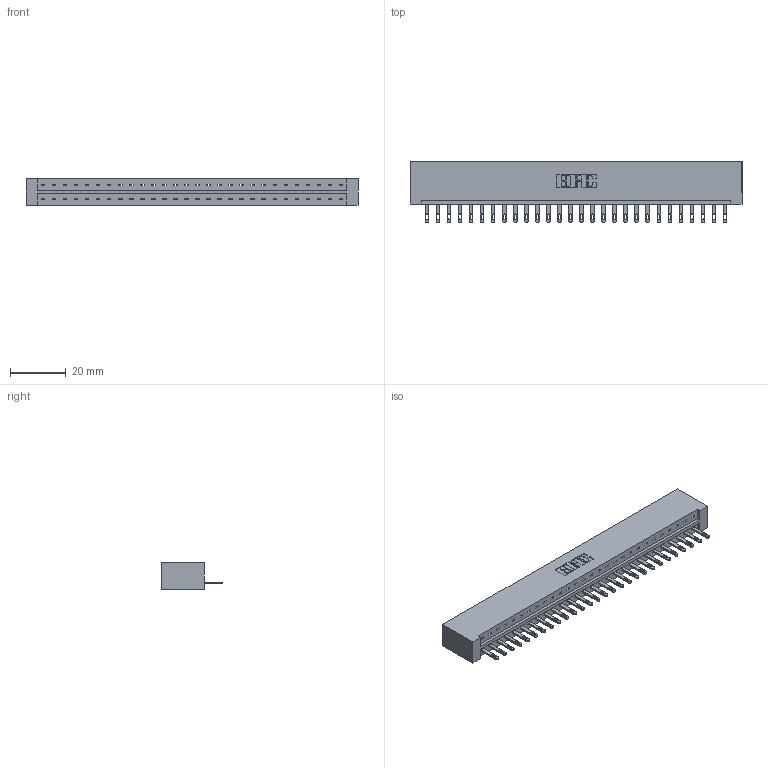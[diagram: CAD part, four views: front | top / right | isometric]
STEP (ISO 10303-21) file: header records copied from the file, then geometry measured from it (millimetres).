
FILE_DESCRIPTION (( 'STEP AP203' ), '1' );
FILE_NAME ('833-028-500-101.STEP', '2020-06-02T07:21:20', ( '' ), ( '' ), 'SwSTEP 2.0', 'SolidWorks 2020', '' );
FILE_SCHEMA (( 'CONFIG_CONTROL_DESIGN' ));
Length unit declared in the file: inch
Products named in the file (3): 833 Part_Lugless; 345-292-001_345-293-100; 833-028-500-101
Assembly tree (29 placements, depth 2):
  833-028-500-101
    833 Part_Lugless
    345-292-001_345-293-100  x28
Bounding box: 119.2 x 21.85 x 9.4 mm (x, y, z)
Volume: 12504.8 mm3; surface area: 13462.9 mm2
Topology: 29 solids, 29 shells, 1618 faces, 4991 edges, 3326 vertices
Faces by surface type: plane 1074, cylinder 544
Entity records: 18581 total; most frequent: CARTESIAN_POINT 3214, ORIENTED_EDGE 3178, DIRECTION 2733, EDGE_CURVE 1589, LINE 1465, VECTOR 1465, VERTEX_POINT 1058, AXIS2_PLACEMENT_3D 634
